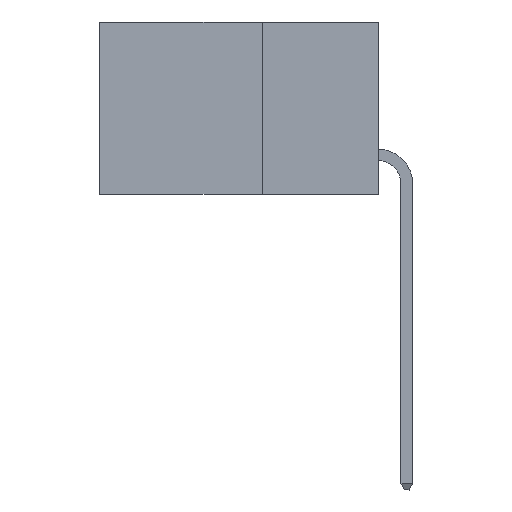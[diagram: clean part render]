
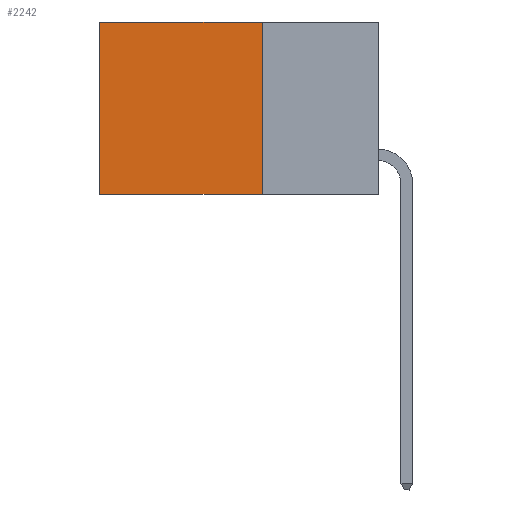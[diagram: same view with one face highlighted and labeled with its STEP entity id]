
A CAD part, left-side view. The second image highlights one B-rep face of the part: STEP entity #2242.
In plain terms, the highlighted planar face has unit normal (-1, 0, 0).
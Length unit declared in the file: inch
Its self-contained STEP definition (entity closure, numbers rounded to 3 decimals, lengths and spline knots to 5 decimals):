
#1156 = LINE ( 'NONE', #8470, #17867 ) ;
#1977 = VERTEX_POINT ( 'NONE', #18121 ) ;
#2242 = ADVANCED_FACE ( 'NONE', ( #20165 ), #15515, .F. ) ;
#2249 = DIRECTION ( 'NONE',  ( 0., 1., 0. ) ) ;
#2254 = ORIENTED_EDGE ( 'NONE', *, *, #23765, .T. ) ;
#2638 = CARTESIAN_POINT ( 'NONE',  ( 0.298, 0.25, -0.37 ) ) ;
#5068 = DIRECTION ( 'NONE',  ( 0., 0., -1. ) ) ;
#5782 = DIRECTION ( 'NONE',  ( 0., 1., 0. ) ) ;
#5971 = CARTESIAN_POINT ( 'NONE',  ( 0.298, 0.25, -0.37 ) ) ;
#6034 = EDGE_CURVE ( 'NONE', #1977, #24656, #9945, .T. ) ;
#7171 = VERTEX_POINT ( 'NONE', #9699 ) ;
#8470 = CARTESIAN_POINT ( 'NONE',  ( 0.298, 0.6, 0. ) ) ;
#9699 = CARTESIAN_POINT ( 'NONE',  ( 0.298, 0.6, -0.37 ) ) ;
#9945 = LINE ( 'NONE', #18445, #26626 ) ;
#12219 = VECTOR ( 'NONE', #5782, 39.37008 ) ;
#12319 = EDGE_CURVE ( 'NONE', #24656, #7171, #24126, .T. ) ;
#14941 = DIRECTION ( 'NONE',  ( 0., 0., -1. ) ) ;
#15515 = PLANE ( 'NONE',  #23659 ) ;
#16481 = EDGE_CURVE ( 'NONE', #21330, #7171, #1156, .T. ) ;
#17095 = CARTESIAN_POINT ( 'NONE',  ( 0.298, 0.25, 0. ) ) ;
#17867 = VECTOR ( 'NONE', #14941, 39.37008 ) ;
#18121 = CARTESIAN_POINT ( 'NONE',  ( 0.298, 0.25, 0. ) ) ;
#18410 = ORIENTED_EDGE ( 'NONE', *, *, #16481, .T. ) ;
#18445 = CARTESIAN_POINT ( 'NONE',  ( 0.298, 0.25, 0. ) ) ;
#19797 = CARTESIAN_POINT ( 'NONE',  ( 0.298, 0.25, 0. ) ) ;
#20165 = FACE_OUTER_BOUND ( 'NONE', #22675, .T. ) ;
#20180 = LINE ( 'NONE', #17095, #26624 ) ;
#21330 = VERTEX_POINT ( 'NONE', #24011 ) ;
#22138 = ORIENTED_EDGE ( 'NONE', *, *, #6034, .F. ) ;
#22675 = EDGE_LOOP ( 'NONE', ( #18410, #28109, #22138, #2254 ) ) ;
#23659 = AXIS2_PLACEMENT_3D ( 'NONE', #19797, #24691, #5068 ) ;
#23765 = EDGE_CURVE ( 'NONE', #1977, #21330, #20180, .T. ) ;
#24011 = CARTESIAN_POINT ( 'NONE',  ( 0.298, 0.6, 0. ) ) ;
#24126 = LINE ( 'NONE', #5971, #12219 ) ;
#24656 = VERTEX_POINT ( 'NONE', #2638 ) ;
#24691 = DIRECTION ( 'NONE',  ( 1., 0., 0. ) ) ;
#26624 = VECTOR ( 'NONE', #2249, 39.37008 ) ;
#26626 = VECTOR ( 'NONE', #27162, 39.37008 ) ;
#27162 = DIRECTION ( 'NONE',  ( 0., 0., -1. ) ) ;
#28109 = ORIENTED_EDGE ( 'NONE', *, *, #12319, .F. ) ;
